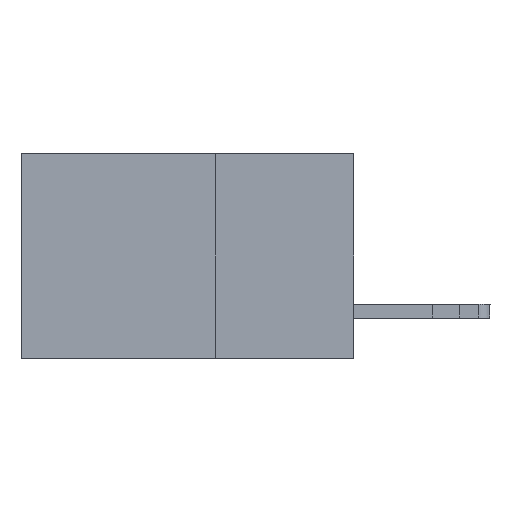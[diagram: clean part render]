
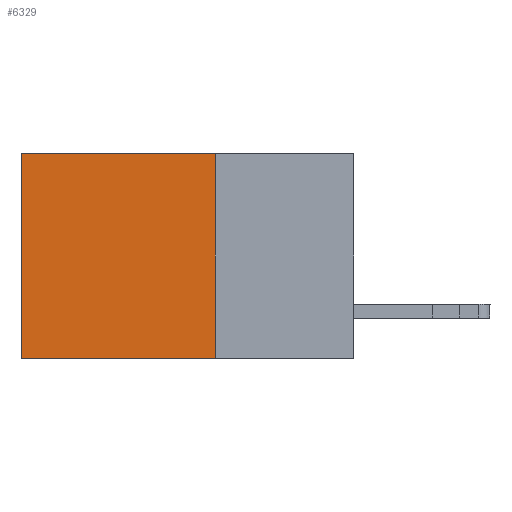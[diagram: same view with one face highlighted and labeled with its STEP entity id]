
A CAD part, left-side view. The second image highlights one B-rep face of the part: STEP entity #6329.
In plain terms, the highlighted planar face has unit normal (-1, 0, 0).
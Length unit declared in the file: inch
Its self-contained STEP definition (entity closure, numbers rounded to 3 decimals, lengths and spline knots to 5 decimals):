
#713 = CARTESIAN_POINT ( 'NONE',  ( 0.2875, 0.25, 0. ) ) ;
#1507 = LINE ( 'NONE', #28945, #4357 ) ;
#1653 = DIRECTION ( 'NONE',  ( 1., 0., 0. ) ) ;
#2554 = DIRECTION ( 'NONE',  ( 0., 0., -1. ) ) ;
#4232 = CARTESIAN_POINT ( 'NONE',  ( 0.2875, 0.6, -0.37 ) ) ;
#4357 = VECTOR ( 'NONE', #8394, 39.37008 ) ;
#5200 = VERTEX_POINT ( 'NONE', #13457 ) ;
#6329 = ADVANCED_FACE ( 'NONE', ( #17557 ), #26699, .F. ) ;
#6489 = EDGE_CURVE ( 'NONE', #5200, #22246, #20550, .T. ) ;
#6549 = EDGE_CURVE ( 'NONE', #27060, #5200, #25928, .T. ) ;
#7575 = ORIENTED_EDGE ( 'NONE', *, *, #19209, .F. ) ;
#7679 = AXIS2_PLACEMENT_3D ( 'NONE', #14710, #1653, #24483 ) ;
#7794 = EDGE_CURVE ( 'NONE', #27060, #8372, #1507, .T. ) ;
#8372 = VERTEX_POINT ( 'NONE', #12629 ) ;
#8394 = DIRECTION ( 'NONE',  ( 0., 0., -1. ) ) ;
#9474 = ORIENTED_EDGE ( 'NONE', *, *, #6489, .T. ) ;
#12005 = LINE ( 'NONE', #27285, #15734 ) ;
#12629 = CARTESIAN_POINT ( 'NONE',  ( 0.2875, 0.25, -0.37 ) ) ;
#13457 = CARTESIAN_POINT ( 'NONE',  ( 0.2875, 0.6, 0. ) ) ;
#14710 = CARTESIAN_POINT ( 'NONE',  ( 0.2875, 0.25, 0. ) ) ;
#15734 = VECTOR ( 'NONE', #25937, 39.37008 ) ;
#17557 = FACE_OUTER_BOUND ( 'NONE', #25330, .T. ) ;
#19209 = EDGE_CURVE ( 'NONE', #8372, #22246, #12005, .T. ) ;
#20550 = LINE ( 'NONE', #27428, #21153 ) ;
#21153 = VECTOR ( 'NONE', #2554, 39.37008 ) ;
#21171 = ORIENTED_EDGE ( 'NONE', *, *, #6549, .T. ) ;
#22246 = VERTEX_POINT ( 'NONE', #4232 ) ;
#24483 = DIRECTION ( 'NONE',  ( 0., 0., -1. ) ) ;
#25303 = ORIENTED_EDGE ( 'NONE', *, *, #7794, .F. ) ;
#25330 = EDGE_LOOP ( 'NONE', ( #9474, #7575, #25303, #21171 ) ) ;
#25928 = LINE ( 'NONE', #713, #28766 ) ;
#25937 = DIRECTION ( 'NONE',  ( 0., 1., 0. ) ) ;
#26493 = CARTESIAN_POINT ( 'NONE',  ( 0.2875, 0.25, 0. ) ) ;
#26699 = PLANE ( 'NONE',  #7679 ) ;
#27060 = VERTEX_POINT ( 'NONE', #26493 ) ;
#27285 = CARTESIAN_POINT ( 'NONE',  ( 0.2875, 0.25, -0.37 ) ) ;
#27428 = CARTESIAN_POINT ( 'NONE',  ( 0.2875, 0.6, 0. ) ) ;
#28135 = DIRECTION ( 'NONE',  ( 0., 1., 0. ) ) ;
#28766 = VECTOR ( 'NONE', #28135, 39.37008 ) ;
#28945 = CARTESIAN_POINT ( 'NONE',  ( 0.2875, 0.25, 0. ) ) ;
